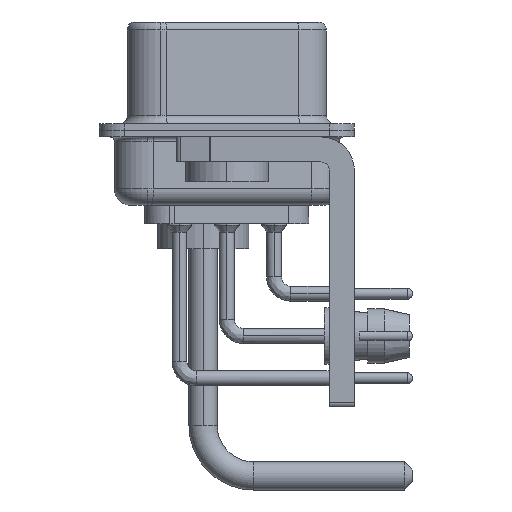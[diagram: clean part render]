
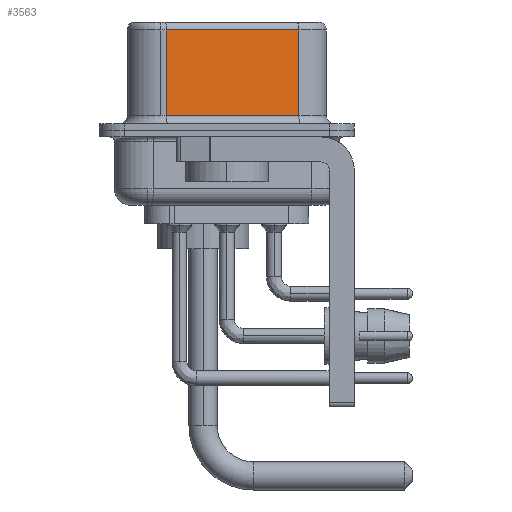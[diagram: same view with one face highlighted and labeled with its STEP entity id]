
A CAD part, left-side view. The second image highlights one B-rep face of the part: STEP entity #3563.
In plain terms, the highlighted planar face has unit normal (-0.985, -0.174, 0).
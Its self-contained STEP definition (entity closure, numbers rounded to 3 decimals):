
#2244 = VERTEX_POINT ( 'NONE', #22747 ) ;
#2726 = LINE ( 'NONE', #15066, #14086 ) ;
#2926 = DIRECTION ( 'NONE',  ( 0., 0., -1. ) ) ;
#2984 = VECTOR ( 'NONE', #19041, 1000. ) ;
#3026 = VERTEX_POINT ( 'NONE', #13344 ) ;
#3563 = ADVANCED_FACE ( 'NONE', ( #5008 ), #35927, .F. ) ;
#5008 = FACE_OUTER_BOUND ( 'NONE', #14336, .T. ) ;
#5400 = CARTESIAN_POINT ( 'NONE',  ( 5.132, -4.322, 6.52 ) ) ;
#6571 = LINE ( 'NONE', #12632, #33347 ) ;
#8601 = EDGE_CURVE ( 'NONE', #17081, #2244, #2726, .T. ) ;
#9000 = DIRECTION ( 'NONE',  ( 0., 0., -1. ) ) ;
#12632 = CARTESIAN_POINT ( 'NONE',  ( 3.73, 3.628, 6.52 ) ) ;
#13344 = CARTESIAN_POINT ( 'NONE',  ( 3.73, 3.628, 0.9 ) ) ;
#13384 = ORIENTED_EDGE ( 'NONE', *, *, #35531, .T. ) ;
#14086 = VECTOR ( 'NONE', #2926, 1000. ) ;
#14336 = EDGE_LOOP ( 'NONE', ( #20756, #24220, #24717, #13384 ) ) ;
#15066 = CARTESIAN_POINT ( 'NONE',  ( 5.132, -4.322, 6.52 ) ) ;
#16601 = CARTESIAN_POINT ( 'NONE',  ( 3.73, 3.628, 6.02 ) ) ;
#17081 = VERTEX_POINT ( 'NONE', #23567 ) ;
#19041 = DIRECTION ( 'NONE',  ( 0.174, -0.985, 0. ) ) ;
#19443 = LINE ( 'NONE', #31973, #22992 ) ;
#20162 = DIRECTION ( 'NONE',  ( 0.985, 0.174, 0. ) ) ;
#20756 = ORIENTED_EDGE ( 'NONE', *, *, #8601, .F. ) ;
#21676 = LINE ( 'NONE', #34217, #2984 ) ;
#22747 = CARTESIAN_POINT ( 'NONE',  ( 5.132, -4.322, 0.9 ) ) ;
#22992 = VECTOR ( 'NONE', #31567, 1000. ) ;
#23213 = DIRECTION ( 'NONE',  ( -0.174, 0.985, 0. ) ) ;
#23567 = CARTESIAN_POINT ( 'NONE',  ( 5.132, -4.322, 6.02 ) ) ;
#24220 = ORIENTED_EDGE ( 'NONE', *, *, #35835, .T. ) ;
#24717 = ORIENTED_EDGE ( 'NONE', *, *, #31952, .T. ) ;
#28068 = AXIS2_PLACEMENT_3D ( 'NONE', #5400, #20162, #23213 ) ;
#31391 = VERTEX_POINT ( 'NONE', #16601 ) ;
#31567 = DIRECTION ( 'NONE',  ( -0.174, 0.985, 0. ) ) ;
#31952 = EDGE_CURVE ( 'NONE', #31391, #3026, #6571, .T. ) ;
#31973 = CARTESIAN_POINT ( 'NONE',  ( 5.132, -4.322, 6.02 ) ) ;
#33347 = VECTOR ( 'NONE', #9000, 1000. ) ;
#34217 = CARTESIAN_POINT ( 'NONE',  ( 5.132, -4.322, 0.9 ) ) ;
#35531 = EDGE_CURVE ( 'NONE', #3026, #2244, #21676, .T. ) ;
#35835 = EDGE_CURVE ( 'NONE', #17081, #31391, #19443, .T. ) ;
#35927 = PLANE ( 'NONE',  #28068 ) ;
